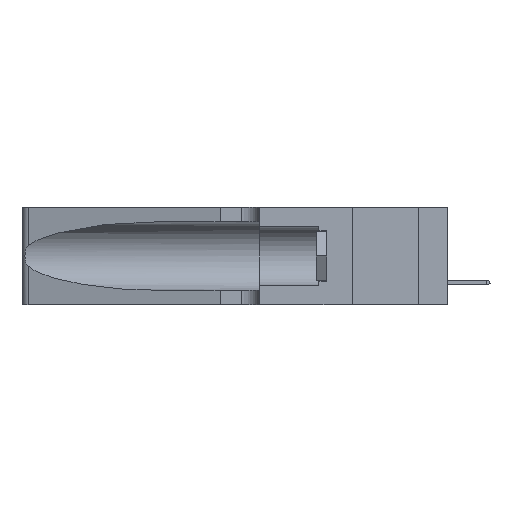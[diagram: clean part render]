
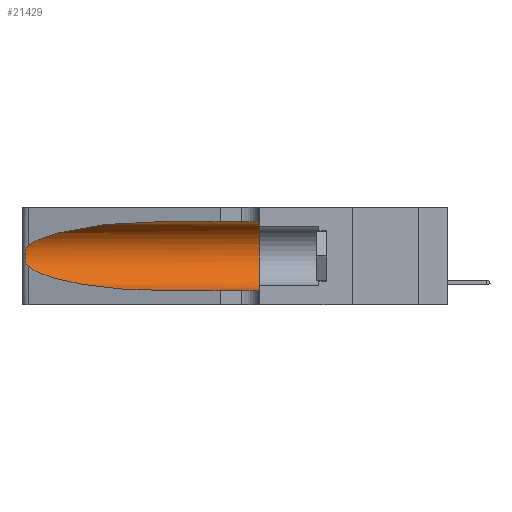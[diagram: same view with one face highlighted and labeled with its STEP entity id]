
A CAD part, left-side view. The second image highlights one B-rep face of the part: STEP entity #21429.
In plain terms, the highlighted cylindrical face has radius 3.308 mm (diameter 6.617 mm), a partial arc.
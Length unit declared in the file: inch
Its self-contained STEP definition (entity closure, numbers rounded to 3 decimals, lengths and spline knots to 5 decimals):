
#1750 = EDGE_CURVE ( 'NONE', #10517, #32722, #31743, .T. ) ;
#1811 = CARTESIAN_POINT ( 'NONE',  ( 0.25487, 1.22718, 0.14631 ) ) ;
#1937 = VERTEX_POINT ( 'NONE', #21415 ) ;
#1984 = EDGE_CURVE ( 'NONE', #1937, #7447, #20305, .T. ) ;
#2736 = DIRECTION ( 'NONE',  ( 0., 0., 1. ) ) ;
#3210 = CARTESIAN_POINT ( 'NONE',  ( 0.18966, 0.96281, 0.31525 ) ) ;
#3825 = DIRECTION ( 'NONE',  ( 0., -1., 0. ) ) ;
#4629 = CARTESIAN_POINT ( 'NONE',  ( 0.25487, 1.22718, 0.14631 ) ) ;
#5214 = CARTESIAN_POINT ( 'NONE',  ( 0.1305, 0.35, 0.31525 ) ) ;
#5223 =( BOUNDED_CURVE ( )  B_SPLINE_CURVE ( 3, ( #26511, #3210, #29939, #21529 ),
 .UNSPECIFIED., .F., .T. ) 
 B_SPLINE_CURVE_WITH_KNOTS ( ( 4, 4 ),
 ( 1.5708, 2.84003 ),
 .UNSPECIFIED. ) 
 CURVE ( )  GEOMETRIC_REPRESENTATION_ITEM ( )  RATIONAL_B_SPLINE_CURVE ( ( 1., 0.87, 0.87, 1. ) ) 
 REPRESENTATION_ITEM ( '' )  );
#5439 = VERTEX_POINT ( 'NONE', #12129 ) ;
#5608 = CARTESIAN_POINT ( 'NONE',  ( 0.25787, 1.23484, 0.2124 ) ) ;
#6414 = CIRCLE ( 'NONE', #9990, 0.13025 ) ;
#6545 = CARTESIAN_POINT ( 'NONE',  ( 0.1305, 1.61858, 0.31525 ) ) ;
#7447 = VERTEX_POINT ( 'NONE', #5214 ) ;
#8108 = EDGE_CURVE ( 'NONE', #1937, #32489, #5223, .T. ) ;
#8448 = VECTOR ( 'NONE', #19517, 39.37008 ) ;
#8921 = EDGE_CURVE ( 'NONE', #32489, #10517, #29828, .T. ) ;
#9990 = AXIS2_PLACEMENT_3D ( 'NONE', #14448, #20431, #2736 ) ;
#10334 = ORIENTED_EDGE ( 'NONE', *, *, #1750, .T. ) ;
#10517 = VERTEX_POINT ( 'NONE', #1811 ) ;
#10600 = AXIS2_PLACEMENT_3D ( 'NONE', #30431, #15264, #19840 ) ;
#12129 = CARTESIAN_POINT ( 'NONE',  ( 0.1305, 0.35, 0.05475 ) ) ;
#12978 = CARTESIAN_POINT ( 'NONE',  ( 0.1305, 0.72297, 0.05475 ) ) ;
#13563 = CARTESIAN_POINT ( 'NONE',  ( 0.1305, 0.72297, 0.05475 ) ) ;
#14348 = CARTESIAN_POINT ( 'NONE',  ( 0.25555, 1.22994, 0.2215 ) ) ;
#14448 = CARTESIAN_POINT ( 'NONE',  ( 0.1305, 0.35, 0.185 ) ) ;
#15030 = EDGE_LOOP ( 'NONE', ( #31320, #26942, #10334, #20417, #15707, #24927 ) ) ;
#15067 = CARTESIAN_POINT ( 'NONE',  ( 0.26075, 1.23896, 0.178 ) ) ;
#15194 = CARTESIAN_POINT ( 'NONE',  ( 0.25856, 1.23593, 0.16098 ) ) ;
#15264 = DIRECTION ( 'NONE',  ( 0., -1., 0. ) ) ;
#15707 = ORIENTED_EDGE ( 'NONE', *, *, #26592, .F. ) ;
#17531 = EDGE_CURVE ( 'NONE', #32722, #5439, #29257, .T. ) ;
#19336 = VECTOR ( 'NONE', #3825, 39.37008 ) ;
#19517 = DIRECTION ( 'NONE',  ( 0., -1., 0. ) ) ;
#19840 = DIRECTION ( 'NONE',  ( 0., 0., -1. ) ) ;
#20086 = CARTESIAN_POINT ( 'NONE',  ( 0.2373, 1.15595, 0.08982 ) ) ;
#20305 = LINE ( 'NONE', #6545, #19336 ) ;
#20417 = ORIENTED_EDGE ( 'NONE', *, *, #17531, .T. ) ;
#20431 = DIRECTION ( 'NONE',  ( 0., 1., 0. ) ) ;
#21321 = CARTESIAN_POINT ( 'NONE',  ( 0.26017, 1.23833, 0.17102 ) ) ;
#21415 = CARTESIAN_POINT ( 'NONE',  ( 0.1305, 0.72297, 0.31525 ) ) ;
#21429 = ADVANCED_FACE ( 'NONE', ( #25281 ), #29394, .F. ) ;
#21529 = CARTESIAN_POINT ( 'NONE',  ( 0.25487, 1.22718, 0.22369 ) ) ;
#23456 = CARTESIAN_POINT ( 'NONE',  ( 0.26018, 1.23835, 0.19895 ) ) ;
#24058 = CARTESIAN_POINT ( 'NONE',  ( 0.25639, 1.23186, 0.15144 ) ) ;
#24172 = CARTESIAN_POINT ( 'NONE',  ( 0.25555, 1.22993, 0.14849 ) ) ;
#24927 = ORIENTED_EDGE ( 'NONE', *, *, #1984, .F. ) ;
#25281 = FACE_OUTER_BOUND ( 'NONE', #15030, .T. ) ;
#25406 = CARTESIAN_POINT ( 'NONE',  ( 0.1305, 1.61858, 0.05475 ) ) ;
#25970 = CARTESIAN_POINT ( 'NONE',  ( 0.25487, 1.22718, 0.22369 ) ) ;
#26302 = CARTESIAN_POINT ( 'NONE',  ( 0.25854, 1.2359, 0.20912 ) ) ;
#26511 = CARTESIAN_POINT ( 'NONE',  ( 0.1305, 0.72297, 0.31525 ) ) ;
#26592 = EDGE_CURVE ( 'NONE', #7447, #5439, #6414, .T. ) ;
#26942 = ORIENTED_EDGE ( 'NONE', *, *, #8921, .T. ) ;
#27267 = CARTESIAN_POINT ( 'NONE',  ( 0.25487, 1.22718, 0.14631 ) ) ;
#29257 = LINE ( 'NONE', #25406, #8448 ) ;
#29394 = CYLINDRICAL_SURFACE ( 'NONE', #10600, 0.13025 ) ;
#29828 = B_SPLINE_CURVE_WITH_KNOTS ( 'NONE', 3,
 ( #34699, #14348, #38010, #5608, #26302, #23456, #36127, #15067, #21321, #15194, #35762, #24058, #24172, #27267 ),
 .UNSPECIFIED., .F., .F.,
 ( 4, 2, 2, 2, 2, 2, 4 ),
 ( 0., 0.00027, 0.00053, 0.00107, 0.0016, 0.00187, 0.00214 ),
 .UNSPECIFIED. ) ;
#29939 = CARTESIAN_POINT ( 'NONE',  ( 0.2373, 1.15595, 0.28018 ) ) ;
#30431 = CARTESIAN_POINT ( 'NONE',  ( 0.1305, 1.61858, 0.185 ) ) ;
#31320 = ORIENTED_EDGE ( 'NONE', *, *, #8108, .T. ) ;
#31743 =( BOUNDED_CURVE ( )  B_SPLINE_CURVE ( 3, ( #4629, #20086, #32908, #13563 ),
 .UNSPECIFIED., .F., .T. ) 
 B_SPLINE_CURVE_WITH_KNOTS ( ( 4, 4 ),
 ( 3.44316, 4.71239 ),
 .UNSPECIFIED. ) 
 CURVE ( )  GEOMETRIC_REPRESENTATION_ITEM ( )  RATIONAL_B_SPLINE_CURVE ( ( 1., 0.87, 0.87, 1. ) ) 
 REPRESENTATION_ITEM ( '' )  );
#32489 = VERTEX_POINT ( 'NONE', #25970 ) ;
#32722 = VERTEX_POINT ( 'NONE', #12978 ) ;
#32908 = CARTESIAN_POINT ( 'NONE',  ( 0.18966, 0.96281, 0.05475 ) ) ;
#34699 = CARTESIAN_POINT ( 'NONE',  ( 0.25487, 1.22718, 0.22369 ) ) ;
#35762 = CARTESIAN_POINT ( 'NONE',  ( 0.25789, 1.23486, 0.15765 ) ) ;
#36127 = CARTESIAN_POINT ( 'NONE',  ( 0.26075, 1.23896, 0.19203 ) ) ;
#38010 = CARTESIAN_POINT ( 'NONE',  ( 0.25639, 1.23184, 0.21858 ) ) ;
